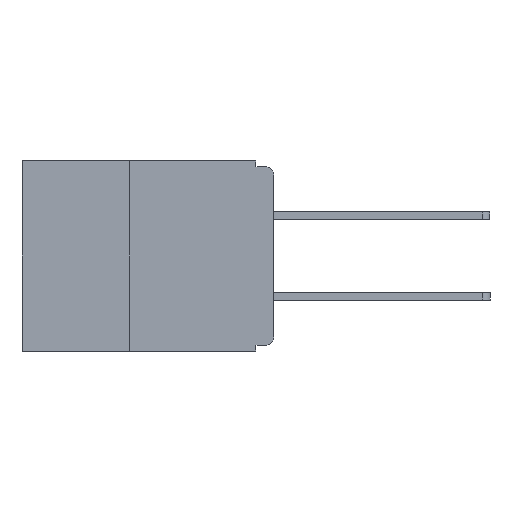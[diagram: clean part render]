
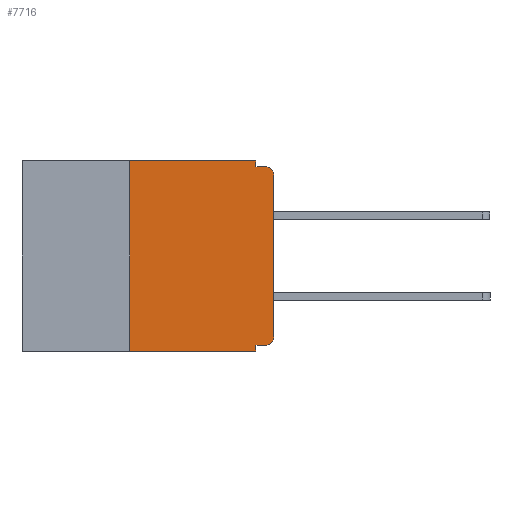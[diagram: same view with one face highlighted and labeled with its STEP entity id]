
A CAD part, left-side view. The second image highlights one B-rep face of the part: STEP entity #7716.
In plain terms, the highlighted planar face has unit normal (-1, 0, 0).
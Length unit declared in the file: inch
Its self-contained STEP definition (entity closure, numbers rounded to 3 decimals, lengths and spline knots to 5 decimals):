
#476 = ORIENTED_EDGE ( 'NONE', *, *, #23263, .T. ) ;
#658 = LINE ( 'NONE', #4877, #24400 ) ;
#976 = ORIENTED_EDGE ( 'NONE', *, *, #1144, .F. ) ;
#1128 = CARTESIAN_POINT ( 'NONE',  ( 0., 0.031, 0. ) ) ;
#1144 = EDGE_CURVE ( 'NONE', #3726, #23046, #7165, .T. ) ;
#2399 = EDGE_CURVE ( 'NONE', #23046, #12440, #9687, .T. ) ;
#2439 = PLANE ( 'NONE',  #10143 ) ;
#2481 = CARTESIAN_POINT ( 'NONE',  ( 0., 0.031, -0.32 ) ) ;
#2596 = EDGE_CURVE ( 'NONE', #20737, #5472, #4593, .T. ) ;
#2892 = AXIS2_PLACEMENT_3D ( 'NONE', #19479, #5672, #21765 ) ;
#3233 = DIRECTION ( 'NONE',  ( 0., -1., 0. ) ) ;
#3606 = VERTEX_POINT ( 'NONE', #2481 ) ;
#3726 = VERTEX_POINT ( 'NONE', #29503 ) ;
#4240 = VECTOR ( 'NONE', #10338, 39.37008 ) ;
#4593 = CIRCLE ( 'NONE', #28978, 0.015 ) ;
#4812 = DIRECTION ( 'NONE',  ( 0., 0., -1. ) ) ;
#4871 = CARTESIAN_POINT ( 'NONE',  ( 0., 0., -0.305 ) ) ;
#4877 = CARTESIAN_POINT ( 'NONE',  ( 0., 0.25, -0.33 ) ) ;
#5135 = CARTESIAN_POINT ( 'NONE',  ( 0., 0., -0.01 ) ) ;
#5472 = VERTEX_POINT ( 'NONE', #4871 ) ;
#5672 = DIRECTION ( 'NONE',  ( -1., 0., 0. ) ) ;
#7165 = LINE ( 'NONE', #20896, #24754 ) ;
#7353 = CARTESIAN_POINT ( 'NONE',  ( 0., 0., -0.32 ) ) ;
#7643 = CARTESIAN_POINT ( 'NONE',  ( 0., 0., -0.025 ) ) ;
#7716 = ADVANCED_FACE ( 'NONE', ( #25195 ), #2439, .F. ) ;
#7734 = CARTESIAN_POINT ( 'NONE',  ( 0., 0.015, -0.01 ) ) ;
#8315 = CARTESIAN_POINT ( 'NONE',  ( 0., 0.25, -0.33 ) ) ;
#9687 = LINE ( 'NONE', #1128, #4240 ) ;
#9794 = ORIENTED_EDGE ( 'NONE', *, *, #2596, .T. ) ;
#9954 = LINE ( 'NONE', #5135, #16062 ) ;
#10143 = AXIS2_PLACEMENT_3D ( 'NONE', #25372, #18644, #4812 ) ;
#10181 = EDGE_CURVE ( 'NONE', #27120, #3726, #658, .T. ) ;
#10338 = DIRECTION ( 'NONE',  ( 0., 0., -1. ) ) ;
#10906 = CARTESIAN_POINT ( 'NONE',  ( 0., 0.031, -0.33 ) ) ;
#11354 = ORIENTED_EDGE ( 'NONE', *, *, #13046, .T. ) ;
#11593 = DIRECTION ( 'NONE',  ( -1., 0., 0. ) ) ;
#11736 = DIRECTION ( 'NONE',  ( 0., 0., -1. ) ) ;
#12440 = VERTEX_POINT ( 'NONE', #28720 ) ;
#12906 = DIRECTION ( 'NONE',  ( 0., 0., -1. ) ) ;
#13046 = EDGE_CURVE ( 'NONE', #5472, #14877, #24256, .T. ) ;
#13542 = CARTESIAN_POINT ( 'NONE',  ( 0., 0.031, 0. ) ) ;
#14758 = CARTESIAN_POINT ( 'NONE',  ( 0., 0.437, -0.33 ) ) ;
#14877 = VERTEX_POINT ( 'NONE', #7643 ) ;
#14941 = CARTESIAN_POINT ( 'NONE',  ( 0., 0., 0. ) ) ;
#15319 = EDGE_LOOP ( 'NONE', ( #11354, #476, #16786, #28612, #976, #26861, #24547, #15337, #28273, #9794 ) ) ;
#15337 = ORIENTED_EDGE ( 'NONE', *, *, #20964, .F. ) ;
#16062 = VECTOR ( 'NONE', #21249, 39.37008 ) ;
#16263 = LINE ( 'NONE', #26583, #21645 ) ;
#16420 = CIRCLE ( 'NONE', #2892, 0.015 ) ;
#16632 = DIRECTION ( 'NONE',  ( 0., 1., 0. ) ) ;
#16769 = VERTEX_POINT ( 'NONE', #10906 ) ;
#16786 = ORIENTED_EDGE ( 'NONE', *, *, #28338, .F. ) ;
#16856 = VECTOR ( 'NONE', #16632, 39.37008 ) ;
#17102 = EDGE_CURVE ( 'NONE', #20737, #3606, #18340, .T. ) ;
#17924 = EDGE_CURVE ( 'NONE', #27120, #16769, #23279, .T. ) ;
#18340 = LINE ( 'NONE', #7353, #16856 ) ;
#18644 = DIRECTION ( 'NONE',  ( 1., 0., 0. ) ) ;
#19479 = CARTESIAN_POINT ( 'NONE',  ( 0., 0.015, -0.025 ) ) ;
#20720 = DIRECTION ( 'NONE',  ( 0., -1., 0. ) ) ;
#20737 = VERTEX_POINT ( 'NONE', #20752 ) ;
#20752 = CARTESIAN_POINT ( 'NONE',  ( 0., 0.015, -0.32 ) ) ;
#20896 = CARTESIAN_POINT ( 'NONE',  ( 0., 0.437, 0. ) ) ;
#20964 = EDGE_CURVE ( 'NONE', #3606, #16769, #16263, .T. ) ;
#20984 = DIRECTION ( 'NONE',  ( 0., 0., 1. ) ) ;
#21249 = DIRECTION ( 'NONE',  ( 0., -1., 0. ) ) ;
#21446 = VERTEX_POINT ( 'NONE', #7734 ) ;
#21645 = VECTOR ( 'NONE', #12906, 39.37008 ) ;
#21765 = DIRECTION ( 'NONE',  ( 0., 0., -1. ) ) ;
#21846 = VECTOR ( 'NONE', #3233, 39.37008 ) ;
#22981 = CARTESIAN_POINT ( 'NONE',  ( 0., 0.015, -0.305 ) ) ;
#23046 = VERTEX_POINT ( 'NONE', #13542 ) ;
#23263 = EDGE_CURVE ( 'NONE', #14877, #21446, #16420, .T. ) ;
#23279 = LINE ( 'NONE', #14758, #21846 ) ;
#24256 = LINE ( 'NONE', #14941, #29549 ) ;
#24400 = VECTOR ( 'NONE', #20984, 39.37008 ) ;
#24547 = ORIENTED_EDGE ( 'NONE', *, *, #17924, .T. ) ;
#24754 = VECTOR ( 'NONE', #20720, 39.37008 ) ;
#25195 = FACE_OUTER_BOUND ( 'NONE', #15319, .T. ) ;
#25372 = CARTESIAN_POINT ( 'NONE',  ( 0., 0.437, 0. ) ) ;
#26583 = CARTESIAN_POINT ( 'NONE',  ( 0., 0.031, -0.33 ) ) ;
#26861 = ORIENTED_EDGE ( 'NONE', *, *, #10181, .F. ) ;
#27120 = VERTEX_POINT ( 'NONE', #8315 ) ;
#28273 = ORIENTED_EDGE ( 'NONE', *, *, #17102, .F. ) ;
#28338 = EDGE_CURVE ( 'NONE', #12440, #21446, #9954, .T. ) ;
#28583 = DIRECTION ( 'NONE',  ( 0., 0., 1. ) ) ;
#28612 = ORIENTED_EDGE ( 'NONE', *, *, #2399, .F. ) ;
#28720 = CARTESIAN_POINT ( 'NONE',  ( 0., 0.031, -0.01 ) ) ;
#28978 = AXIS2_PLACEMENT_3D ( 'NONE', #22981, #11593, #11736 ) ;
#29503 = CARTESIAN_POINT ( 'NONE',  ( 0., 0.25, 0. ) ) ;
#29549 = VECTOR ( 'NONE', #28583, 39.37008 ) ;
